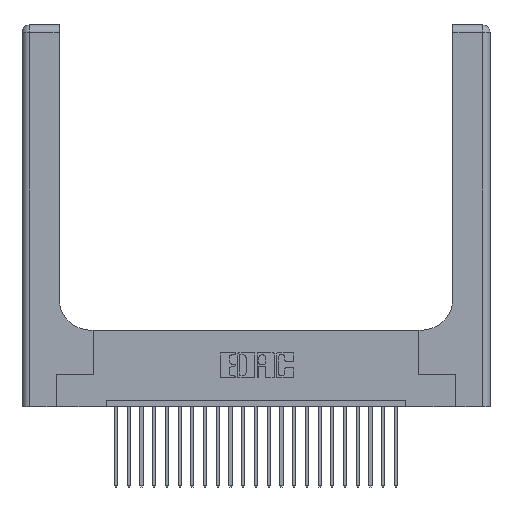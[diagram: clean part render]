
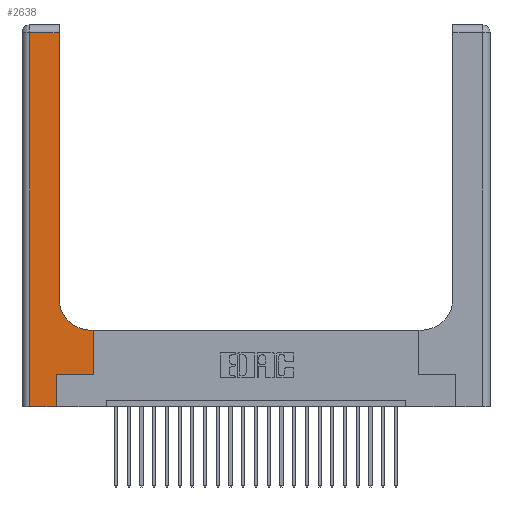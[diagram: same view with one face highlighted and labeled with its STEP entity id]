
A CAD part, top view. The second image highlights one B-rep face of the part: STEP entity #2638.
In plain terms, the highlighted planar face has unit normal (0, 0, 1).
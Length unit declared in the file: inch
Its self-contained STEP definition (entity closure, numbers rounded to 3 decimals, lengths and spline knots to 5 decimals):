
#153 = VECTOR ( 'NONE', #16283, 39.37008 ) ;
#1521 = EDGE_LOOP ( 'NONE', ( #15602, #19997, #8971, #12933, #20976, #16745, #23972, #20222, #11451 ) ) ;
#1662 = LINE ( 'NONE', #22754, #5063 ) ;
#1718 = VERTEX_POINT ( 'NONE', #22422 ) ;
#2172 = CARTESIAN_POINT ( 'NONE',  ( 0.06, 3., 0.37 ) ) ;
#2209 = VERTEX_POINT ( 'NONE', #19328 ) ;
#2240 = CARTESIAN_POINT ( 'NONE',  ( 0.5415, 0.85, 0.37 ) ) ;
#2249 = CIRCLE ( 'NONE', #21530, 0.25 ) ;
#2255 = DIRECTION ( 'NONE',  ( 0., -1., 0. ) ) ;
#2374 = CARTESIAN_POINT ( 'NONE',  ( 0.06, 2.94, 0.37 ) ) ;
#2638 = ADVANCED_FACE ( 'NONE', ( #17452 ), #2930, .F. ) ;
#2643 = CARTESIAN_POINT ( 'NONE',  ( 0., 0., 0.37 ) ) ;
#2734 = LINE ( 'NONE', #2172, #19142 ) ;
#2830 = LINE ( 'NONE', #8923, #15619 ) ;
#2835 = EDGE_CURVE ( 'NONE', #5178, #15767, #2830, .T. ) ;
#2854 = CARTESIAN_POINT ( 'NONE',  ( 0.2915, 2.94, 0.37 ) ) ;
#2930 = PLANE ( 'NONE',  #13925 ) ;
#4143 = DIRECTION ( 'NONE',  ( 0., 0., -1. ) ) ;
#4645 = VERTEX_POINT ( 'NONE', #2854 ) ;
#5063 = VECTOR ( 'NONE', #11200, 39.37008 ) ;
#5178 = VERTEX_POINT ( 'NONE', #9637 ) ;
#5438 = DIRECTION ( 'NONE',  ( -1., 0., 0. ) ) ;
#5518 = DIRECTION ( 'NONE',  ( 1., 0., 0. ) ) ;
#5655 = EDGE_CURVE ( 'NONE', #15767, #18369, #14543, .T. ) ;
#6033 = LINE ( 'NONE', #20689, #19016 ) ;
#6149 = DIRECTION ( 'NONE',  ( 1., 0., 0. ) ) ;
#6857 = DIRECTION ( 'NONE',  ( -1., 0., 0. ) ) ;
#8273 = CARTESIAN_POINT ( 'NONE',  ( 0.5415, 0.6, 0.37 ) ) ;
#8916 = CARTESIAN_POINT ( 'NONE',  ( 0.2915, 0.85, 0.37 ) ) ;
#8923 = CARTESIAN_POINT ( 'NONE',  ( 0.5585, 0.25, 0.37 ) ) ;
#8971 = ORIENTED_EDGE ( 'NONE', *, *, #24942, .T. ) ;
#9171 = CARTESIAN_POINT ( 'NONE',  ( 0.269, 0.25, 0.37 ) ) ;
#9637 = CARTESIAN_POINT ( 'NONE',  ( 0.5585, 0.25, 0.37 ) ) ;
#9680 = DIRECTION ( 'NONE',  ( 0., 1., 0. ) ) ;
#10943 = CARTESIAN_POINT ( 'NONE',  ( 0., 3., 0.37 ) ) ;
#11200 = DIRECTION ( 'NONE',  ( 0., 1., 0. ) ) ;
#11451 = ORIENTED_EDGE ( 'NONE', *, *, #20554, .T. ) ;
#11873 = CARTESIAN_POINT ( 'NONE',  ( 0.2915, 3., 0.37 ) ) ;
#12063 = VECTOR ( 'NONE', #5518, 39.37008 ) ;
#12933 = ORIENTED_EDGE ( 'NONE', *, *, #15618, .T. ) ;
#13908 = EDGE_CURVE ( 'NONE', #22577, #4645, #16068, .T. ) ;
#13925 = AXIS2_PLACEMENT_3D ( 'NONE', #10943, #22435, #24420 ) ;
#14543 = LINE ( 'NONE', #14798, #23837 ) ;
#14798 = CARTESIAN_POINT ( 'NONE',  ( 0.2915, 0.6, 0.37 ) ) ;
#14908 = CARTESIAN_POINT ( 'NONE',  ( 0.5585, 0.6, 0.37 ) ) ;
#15602 = ORIENTED_EDGE ( 'NONE', *, *, #13908, .T. ) ;
#15618 = EDGE_CURVE ( 'NONE', #20721, #2209, #24721, .T. ) ;
#15619 = VECTOR ( 'NONE', #23084, 39.37008 ) ;
#15767 = VERTEX_POINT ( 'NONE', #14908 ) ;
#16067 = EDGE_CURVE ( 'NONE', #2209, #1718, #1662, .T. ) ;
#16068 = LINE ( 'NONE', #11873, #19376 ) ;
#16283 = DIRECTION ( 'NONE',  ( 1., 0., 0. ) ) ;
#16745 = ORIENTED_EDGE ( 'NONE', *, *, #19358, .T. ) ;
#17452 = FACE_OUTER_BOUND ( 'NONE', #1521, .T. ) ;
#18369 = VERTEX_POINT ( 'NONE', #8273 ) ;
#19016 = VECTOR ( 'NONE', #5438, 39.37008 ) ;
#19142 = VECTOR ( 'NONE', #2255, 39.37008 ) ;
#19261 = EDGE_CURVE ( 'NONE', #4645, #21140, #6033, .T. ) ;
#19328 = CARTESIAN_POINT ( 'NONE',  ( 0.269, 0., 0.37 ) ) ;
#19358 = EDGE_CURVE ( 'NONE', #1718, #5178, #21751, .T. ) ;
#19376 = VECTOR ( 'NONE', #9680, 39.37008 ) ;
#19997 = ORIENTED_EDGE ( 'NONE', *, *, #19261, .T. ) ;
#20222 = ORIENTED_EDGE ( 'NONE', *, *, #5655, .T. ) ;
#20554 = EDGE_CURVE ( 'NONE', #18369, #22577, #2249, .T. ) ;
#20689 = CARTESIAN_POINT ( 'NONE',  ( 0., 2.94, 0.37 ) ) ;
#20721 = VERTEX_POINT ( 'NONE', #21373 ) ;
#20976 = ORIENTED_EDGE ( 'NONE', *, *, #16067, .T. ) ;
#21140 = VERTEX_POINT ( 'NONE', #2374 ) ;
#21373 = CARTESIAN_POINT ( 'NONE',  ( 0.06, 0., 0.37 ) ) ;
#21530 = AXIS2_PLACEMENT_3D ( 'NONE', #2240, #4143, #6149 ) ;
#21751 = LINE ( 'NONE', #9171, #12063 ) ;
#22422 = CARTESIAN_POINT ( 'NONE',  ( 0.269, 0.25, 0.37 ) ) ;
#22435 = DIRECTION ( 'NONE',  ( 0., 0., -1. ) ) ;
#22577 = VERTEX_POINT ( 'NONE', #8916 ) ;
#22754 = CARTESIAN_POINT ( 'NONE',  ( 0.269, 0., 0.37 ) ) ;
#23084 = DIRECTION ( 'NONE',  ( 0., 1., 0. ) ) ;
#23837 = VECTOR ( 'NONE', #6857, 39.37008 ) ;
#23972 = ORIENTED_EDGE ( 'NONE', *, *, #2835, .T. ) ;
#24420 = DIRECTION ( 'NONE',  ( -1., 0., 0. ) ) ;
#24721 = LINE ( 'NONE', #2643, #153 ) ;
#24942 = EDGE_CURVE ( 'NONE', #21140, #20721, #2734, .T. ) ;
